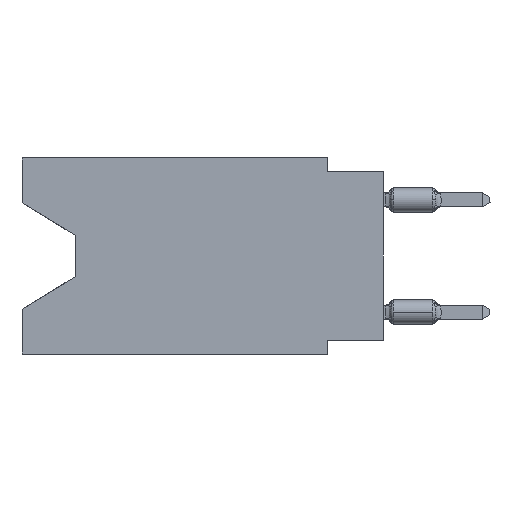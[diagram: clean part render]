
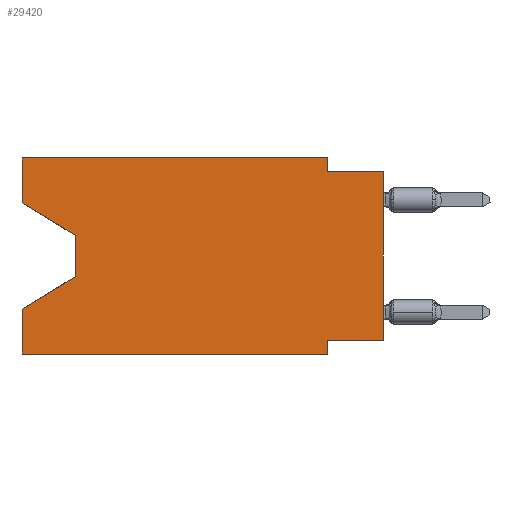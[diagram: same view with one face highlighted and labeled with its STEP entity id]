
A CAD part, left-side view. The second image highlights one B-rep face of the part: STEP entity #29420.
In plain terms, the highlighted planar face has unit normal (-1, 0, 0).
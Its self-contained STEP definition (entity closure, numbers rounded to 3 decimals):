
#66 = VECTOR ( 'NONE', #9362, 1000. ) ;
#395 = ORIENTED_EDGE ( 'NONE', *, *, #26485, .F. ) ;
#674 = LINE ( 'NONE', #3892, #66 ) ;
#1404 = VECTOR ( 'NONE', #33667, 1000. ) ;
#1405 = CARTESIAN_POINT ( 'NONE',  ( 0., 0., -0.635 ) ) ;
#1709 = ORIENTED_EDGE ( 'NONE', *, *, #2996, .T. ) ;
#2346 = CARTESIAN_POINT ( 'NONE',  ( 0., 2.54, -8.255 ) ) ;
#2388 = VECTOR ( 'NONE', #25916, 1000. ) ;
#2996 = EDGE_CURVE ( 'NONE', #15584, #35635, #10853, .T. ) ;
#3114 = CARTESIAN_POINT ( 'NONE',  ( 0., 2.54, 0. ) ) ;
#3892 = CARTESIAN_POINT ( 'NONE',  ( 0., 16.383, 0. ) ) ;
#4212 = VERTEX_POINT ( 'NONE', #3114 ) ;
#4531 = DIRECTION ( 'NONE',  ( 0., 0.855, -0.519 ) ) ;
#5513 = VECTOR ( 'NONE', #22413, 1000. ) ;
#5901 = EDGE_CURVE ( 'NONE', #35635, #9474, #31632, .T. ) ;
#5944 = CARTESIAN_POINT ( 'NONE',  ( 0., 0., -8.255 ) ) ;
#6036 = CARTESIAN_POINT ( 'NONE',  ( 0., 2.54, 0. ) ) ;
#6098 = EDGE_CURVE ( 'NONE', #25285, #12467, #28802, .T. ) ;
#6853 = FACE_OUTER_BOUND ( 'NONE', #27050, .T. ) ;
#7595 = DIRECTION ( 'NONE',  ( 0., -1., 0. ) ) ;
#8108 = CARTESIAN_POINT ( 'NONE',  ( 0., 2.54, -0.635 ) ) ;
#8567 = CARTESIAN_POINT ( 'NONE',  ( 0., 16.383, 0. ) ) ;
#8595 = VERTEX_POINT ( 'NONE', #14377 ) ;
#9362 = DIRECTION ( 'NONE',  ( 0., 0., 1. ) ) ;
#9474 = VERTEX_POINT ( 'NONE', #10432 ) ;
#9937 = VECTOR ( 'NONE', #23130, 1000. ) ;
#10223 = AXIS2_PLACEMENT_3D ( 'NONE', #36110, #33272, #18176 ) ;
#10305 = VECTOR ( 'NONE', #7595, 1000. ) ;
#10370 = LINE ( 'NONE', #24905, #23019 ) ;
#10432 = CARTESIAN_POINT ( 'NONE',  ( 0., 13.97, -5.385 ) ) ;
#10853 = LINE ( 'NONE', #16898, #17133 ) ;
#10889 = LINE ( 'NONE', #5944, #5513 ) ;
#11242 = ORIENTED_EDGE ( 'NONE', *, *, #29268, .T. ) ;
#11438 = EDGE_CURVE ( 'NONE', #4212, #25285, #20392, .T. ) ;
#12467 = VERTEX_POINT ( 'NONE', #1405 ) ;
#12563 = VECTOR ( 'NONE', #25564, 1000. ) ;
#12893 = CARTESIAN_POINT ( 'NONE',  ( 0., 2.54, -8.89 ) ) ;
#13651 = VECTOR ( 'NONE', #17089, 1000. ) ;
#13716 = CARTESIAN_POINT ( 'NONE',  ( 0., 2.54, -8.89 ) ) ;
#13799 = EDGE_CURVE ( 'NONE', #8595, #26404, #14241, .T. ) ;
#14241 = LINE ( 'NONE', #8567, #12563 ) ;
#14377 = CARTESIAN_POINT ( 'NONE',  ( 0., 16.383, -8.89 ) ) ;
#14672 = ORIENTED_EDGE ( 'NONE', *, *, #5901, .T. ) ;
#15584 = VERTEX_POINT ( 'NONE', #30243 ) ;
#15852 = VECTOR ( 'NONE', #33858, 1000. ) ;
#16898 = CARTESIAN_POINT ( 'NONE',  ( 0., 16.383, -2.038 ) ) ;
#17089 = DIRECTION ( 'NONE',  ( 0., 0., -1. ) ) ;
#17133 = VECTOR ( 'NONE', #19364, 1000. ) ;
#17549 = DIRECTION ( 'NONE',  ( 0., 0., -1. ) ) ;
#17580 = VERTEX_POINT ( 'NONE', #13716 ) ;
#17710 = VERTEX_POINT ( 'NONE', #17985 ) ;
#17985 = CARTESIAN_POINT ( 'NONE',  ( 0., 0., -8.255 ) ) ;
#18176 = DIRECTION ( 'NONE',  ( 0., 0., -1. ) ) ;
#18577 = CARTESIAN_POINT ( 'NONE',  ( 0., 16.383, -6.852 ) ) ;
#19364 = DIRECTION ( 'NONE',  ( 0., -0.855, -0.519 ) ) ;
#20392 = LINE ( 'NONE', #6036, #25523 ) ;
#20429 = VERTEX_POINT ( 'NONE', #21796 ) ;
#20575 = ORIENTED_EDGE ( 'NONE', *, *, #26422, .F. ) ;
#21515 = EDGE_CURVE ( 'NONE', #15584, #20429, #674, .T. ) ;
#21796 = CARTESIAN_POINT ( 'NONE',  ( 0., 16.383, 0. ) ) ;
#22058 = ORIENTED_EDGE ( 'NONE', *, *, #30642, .T. ) ;
#22323 = CARTESIAN_POINT ( 'NONE',  ( 0., 16.383, 0. ) ) ;
#22413 = DIRECTION ( 'NONE',  ( 0., 1., 0. ) ) ;
#23019 = VECTOR ( 'NONE', #4531, 1000. ) ;
#23130 = DIRECTION ( 'NONE',  ( 0., -1., 0. ) ) ;
#24905 = CARTESIAN_POINT ( 'NONE',  ( 0., 13.97, -5.385 ) ) ;
#25157 = LINE ( 'NONE', #22323, #15852 ) ;
#25285 = VERTEX_POINT ( 'NONE', #8108 ) ;
#25523 = VECTOR ( 'NONE', #17549, 1000. ) ;
#25564 = DIRECTION ( 'NONE',  ( 0., 0., 1. ) ) ;
#25916 = DIRECTION ( 'NONE',  ( 0., 0., 1. ) ) ;
#25951 = CARTESIAN_POINT ( 'NONE',  ( 0., 0., -0.635 ) ) ;
#26404 = VERTEX_POINT ( 'NONE', #18577 ) ;
#26422 = EDGE_CURVE ( 'NONE', #32063, #17580, #36500, .T. ) ;
#26485 = EDGE_CURVE ( 'NONE', #20429, #4212, #25157, .T. ) ;
#26850 = PLANE ( 'NONE',  #10223 ) ;
#27050 = EDGE_LOOP ( 'NONE', ( #1709, #14672, #34153, #31843, #22058, #20575, #35822, #11242, #37312, #36094, #395, #34745 ) ) ;
#28466 = CARTESIAN_POINT ( 'NONE',  ( 0., 13.97, -3.505 ) ) ;
#28802 = LINE ( 'NONE', #25951, #9937 ) ;
#29268 = EDGE_CURVE ( 'NONE', #17710, #12467, #31969, .T. ) ;
#29420 = ADVANCED_FACE ( 'NONE', ( #6853 ), #26850, .F. ) ;
#30243 = CARTESIAN_POINT ( 'NONE',  ( 0., 16.383, -2.038 ) ) ;
#30642 = EDGE_CURVE ( 'NONE', #8595, #17580, #33470, .T. ) ;
#31632 = LINE ( 'NONE', #37130, #13651 ) ;
#31843 = ORIENTED_EDGE ( 'NONE', *, *, #13799, .F. ) ;
#31969 = LINE ( 'NONE', #35373, #2388 ) ;
#32063 = VERTEX_POINT ( 'NONE', #2346 ) ;
#33272 = DIRECTION ( 'NONE',  ( 1., 0., 0. ) ) ;
#33470 = LINE ( 'NONE', #35939, #10305 ) ;
#33667 = DIRECTION ( 'NONE',  ( 0., 0., -1. ) ) ;
#33858 = DIRECTION ( 'NONE',  ( 0., -1., 0. ) ) ;
#34153 = ORIENTED_EDGE ( 'NONE', *, *, #35243, .T. ) ;
#34582 = EDGE_CURVE ( 'NONE', #17710, #32063, #10889, .T. ) ;
#34745 = ORIENTED_EDGE ( 'NONE', *, *, #21515, .F. ) ;
#35243 = EDGE_CURVE ( 'NONE', #9474, #26404, #10370, .T. ) ;
#35373 = CARTESIAN_POINT ( 'NONE',  ( 0., 0., 0. ) ) ;
#35635 = VERTEX_POINT ( 'NONE', #28466 ) ;
#35822 = ORIENTED_EDGE ( 'NONE', *, *, #34582, .F. ) ;
#35939 = CARTESIAN_POINT ( 'NONE',  ( 0., 16.383, -8.89 ) ) ;
#36094 = ORIENTED_EDGE ( 'NONE', *, *, #11438, .F. ) ;
#36110 = CARTESIAN_POINT ( 'NONE',  ( 0., 16.383, 0. ) ) ;
#36500 = LINE ( 'NONE', #12893, #1404 ) ;
#37130 = CARTESIAN_POINT ( 'NONE',  ( 0., 13.97, -3.505 ) ) ;
#37312 = ORIENTED_EDGE ( 'NONE', *, *, #6098, .F. ) ;
